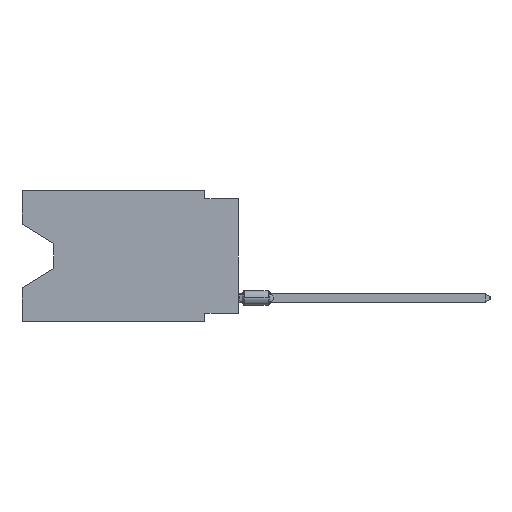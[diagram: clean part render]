
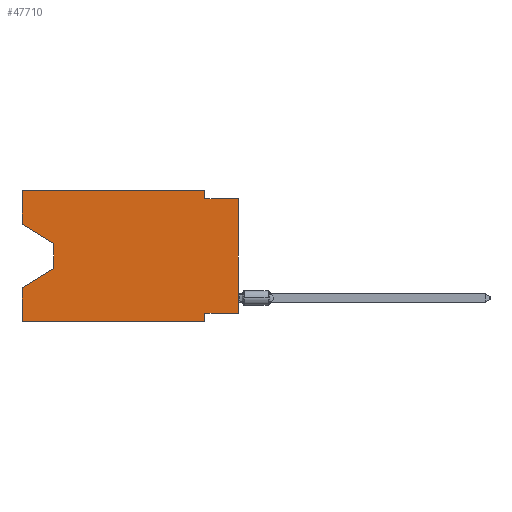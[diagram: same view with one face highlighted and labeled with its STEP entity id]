
A CAD part, left-side view. The second image highlights one B-rep face of the part: STEP entity #47710.
In plain terms, the highlighted planar face has unit normal (-1, 0, 0).
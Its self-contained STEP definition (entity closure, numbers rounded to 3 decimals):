
#558 = EDGE_CURVE ( 'NONE', #9893, #19057, #9636, .T. ) ;
#1325 = EDGE_CURVE ( 'NONE', #52957, #6432, #39212, .T. ) ;
#2985 = EDGE_LOOP ( 'NONE', ( #33727, #47088, #50437, #7218, #51999, #18571, #7102, #35279, #55374, #57346, #28051, #16288 ) ) ;
#3680 = DIRECTION ( 'NONE',  ( 0., -1., 0. ) ) ;
#3991 = CARTESIAN_POINT ( 'NONE',  ( 0., 0., -0.635 ) ) ;
#4182 = CARTESIAN_POINT ( 'NONE',  ( 0., 2.54, -9.906 ) ) ;
#6366 = EDGE_CURVE ( 'NONE', #36349, #51191, #26372, .T. ) ;
#6432 = VERTEX_POINT ( 'NONE', #18864 ) ;
#6901 = LINE ( 'NONE', #19552, #10708 ) ;
#7102 = ORIENTED_EDGE ( 'NONE', *, *, #9890, .F. ) ;
#7218 = ORIENTED_EDGE ( 'NONE', *, *, #42083, .F. ) ;
#9636 = LINE ( 'NONE', #43166, #34267 ) ;
#9775 = EDGE_CURVE ( 'NONE', #51191, #6432, #36428, .T. ) ;
#9890 = EDGE_CURVE ( 'NONE', #52957, #48133, #14819, .T. ) ;
#9893 = VERTEX_POINT ( 'NONE', #28328 ) ;
#10708 = VECTOR ( 'NONE', #52822, 1000. ) ;
#12732 = LINE ( 'NONE', #26252, #39165 ) ;
#14649 = CARTESIAN_POINT ( 'NONE',  ( 0., 16.383, -7.36 ) ) ;
#14790 = EDGE_CURVE ( 'NONE', #48133, #17915, #56411, .T. ) ;
#14819 = LINE ( 'NONE', #32510, #48530 ) ;
#15948 = CARTESIAN_POINT ( 'NONE',  ( 0., 16.383, -9.906 ) ) ;
#16288 = ORIENTED_EDGE ( 'NONE', *, *, #55494, .F. ) ;
#17915 = VERTEX_POINT ( 'NONE', #4182 ) ;
#18571 = ORIENTED_EDGE ( 'NONE', *, *, #14790, .F. ) ;
#18577 = CARTESIAN_POINT ( 'NONE',  ( 0., 16.383, -2.546 ) ) ;
#18864 = CARTESIAN_POINT ( 'NONE',  ( 0., 0., -0.635 ) ) ;
#19057 = VERTEX_POINT ( 'NONE', #14649 ) ;
#19552 = CARTESIAN_POINT ( 'NONE',  ( 0., 16.383, 0. ) ) ;
#19988 = VERTEX_POINT ( 'NONE', #52280 ) ;
#21452 = VECTOR ( 'NONE', #28220, 1000. ) ;
#24285 = DIRECTION ( 'NONE',  ( 0., 0., -1. ) ) ;
#24573 = CARTESIAN_POINT ( 'NONE',  ( 0., 0., -9.271 ) ) ;
#26252 = CARTESIAN_POINT ( 'NONE',  ( 0., 16.383, 0. ) ) ;
#26372 = LINE ( 'NONE', #57882, #40381 ) ;
#26378 = VECTOR ( 'NONE', #57376, 1000. ) ;
#26532 = CARTESIAN_POINT ( 'NONE',  ( 0., 2.54, -0.635 ) ) ;
#27927 = CARTESIAN_POINT ( 'NONE',  ( 0., 2.54, -9.906 ) ) ;
#27998 = VECTOR ( 'NONE', #24285, 1000. ) ;
#28051 = ORIENTED_EDGE ( 'NONE', *, *, #52670, .F. ) ;
#28220 = DIRECTION ( 'NONE',  ( 0., 0., -1. ) ) ;
#28328 = CARTESIAN_POINT ( 'NONE',  ( 0., 13.97, -5.893 ) ) ;
#29158 = VERTEX_POINT ( 'NONE', #18577 ) ;
#30571 = AXIS2_PLACEMENT_3D ( 'NONE', #49865, #44477, #31270 ) ;
#30951 = CARTESIAN_POINT ( 'NONE',  ( 0., 16.383, -9.906 ) ) ;
#31270 = DIRECTION ( 'NONE',  ( 0., 0., -1. ) ) ;
#31559 = FACE_OUTER_BOUND ( 'NONE', #2985, .T. ) ;
#32510 = CARTESIAN_POINT ( 'NONE',  ( 0., 0., -9.271 ) ) ;
#33137 = VERTEX_POINT ( 'NONE', #30951 ) ;
#33569 = CARTESIAN_POINT ( 'NONE',  ( 0., 13.97, -4.013 ) ) ;
#33727 = ORIENTED_EDGE ( 'NONE', *, *, #41891, .T. ) ;
#34267 = VECTOR ( 'NONE', #50456, 1000. ) ;
#34350 = EDGE_CURVE ( 'NONE', #43345, #9893, #53033, .T. ) ;
#35279 = ORIENTED_EDGE ( 'NONE', *, *, #1325, .T. ) ;
#35457 = PLANE ( 'NONE',  #30571 ) ;
#36349 = VERTEX_POINT ( 'NONE', #40175 ) ;
#36428 = LINE ( 'NONE', #3991, #47593 ) ;
#37922 = DIRECTION ( 'NONE',  ( 0., 1., 0. ) ) ;
#38048 = DIRECTION ( 'NONE',  ( 0., 0., 1. ) ) ;
#38494 = CARTESIAN_POINT ( 'NONE',  ( 0., 16.383, -2.546 ) ) ;
#39070 = LINE ( 'NONE', #38494, #26378 ) ;
#39165 = VECTOR ( 'NONE', #40067, 1000. ) ;
#39212 = LINE ( 'NONE', #57507, #58551 ) ;
#40067 = DIRECTION ( 'NONE',  ( 0., 0., 1. ) ) ;
#40175 = CARTESIAN_POINT ( 'NONE',  ( 0., 2.54, 0. ) ) ;
#40381 = VECTOR ( 'NONE', #45284, 1000. ) ;
#41891 = EDGE_CURVE ( 'NONE', #29158, #43345, #39070, .T. ) ;
#42083 = EDGE_CURVE ( 'NONE', #33137, #19057, #56656, .T. ) ;
#43166 = CARTESIAN_POINT ( 'NONE',  ( 0., 13.97, -5.893 ) ) ;
#43345 = VERTEX_POINT ( 'NONE', #52219 ) ;
#44477 = DIRECTION ( 'NONE',  ( 1., 0., 0. ) ) ;
#45284 = DIRECTION ( 'NONE',  ( 0., 0., -1. ) ) ;
#47088 = ORIENTED_EDGE ( 'NONE', *, *, #34350, .T. ) ;
#47593 = VECTOR ( 'NONE', #3680, 1000. ) ;
#47710 = ADVANCED_FACE ( 'NONE', ( #31559 ), #35457, .F. ) ;
#48054 = LINE ( 'NONE', #15948, #49557 ) ;
#48133 = VERTEX_POINT ( 'NONE', #49198 ) ;
#48530 = VECTOR ( 'NONE', #37922, 1000. ) ;
#49198 = CARTESIAN_POINT ( 'NONE',  ( 0., 2.54, -9.271 ) ) ;
#49557 = VECTOR ( 'NONE', #52541, 1000. ) ;
#49865 = CARTESIAN_POINT ( 'NONE',  ( 0., 16.383, 0. ) ) ;
#50437 = ORIENTED_EDGE ( 'NONE', *, *, #558, .T. ) ;
#50456 = DIRECTION ( 'NONE',  ( 0., 0.855, -0.519 ) ) ;
#51191 = VERTEX_POINT ( 'NONE', #26532 ) ;
#51999 = ORIENTED_EDGE ( 'NONE', *, *, #53730, .T. ) ;
#52124 = VECTOR ( 'NONE', #38048, 1000. ) ;
#52219 = CARTESIAN_POINT ( 'NONE',  ( 0., 13.97, -4.013 ) ) ;
#52280 = CARTESIAN_POINT ( 'NONE',  ( 0., 16.383, 0. ) ) ;
#52541 = DIRECTION ( 'NONE',  ( 0., -1., 0. ) ) ;
#52670 = EDGE_CURVE ( 'NONE', #19988, #36349, #6901, .T. ) ;
#52822 = DIRECTION ( 'NONE',  ( 0., -1., 0. ) ) ;
#52957 = VERTEX_POINT ( 'NONE', #24573 ) ;
#53033 = LINE ( 'NONE', #33569, #27998 ) ;
#53730 = EDGE_CURVE ( 'NONE', #33137, #17915, #48054, .T. ) ;
#54184 = DIRECTION ( 'NONE',  ( 0., 0., 1. ) ) ;
#55374 = ORIENTED_EDGE ( 'NONE', *, *, #9775, .F. ) ;
#55494 = EDGE_CURVE ( 'NONE', #29158, #19988, #12732, .T. ) ;
#56358 = CARTESIAN_POINT ( 'NONE',  ( 0., 16.383, 0. ) ) ;
#56411 = LINE ( 'NONE', #27927, #21452 ) ;
#56656 = LINE ( 'NONE', #56358, #52124 ) ;
#57346 = ORIENTED_EDGE ( 'NONE', *, *, #6366, .F. ) ;
#57376 = DIRECTION ( 'NONE',  ( 0., -0.855, -0.519 ) ) ;
#57507 = CARTESIAN_POINT ( 'NONE',  ( 0., 0., 0. ) ) ;
#57882 = CARTESIAN_POINT ( 'NONE',  ( 0., 2.54, 0. ) ) ;
#58551 = VECTOR ( 'NONE', #54184, 1000. ) ;
